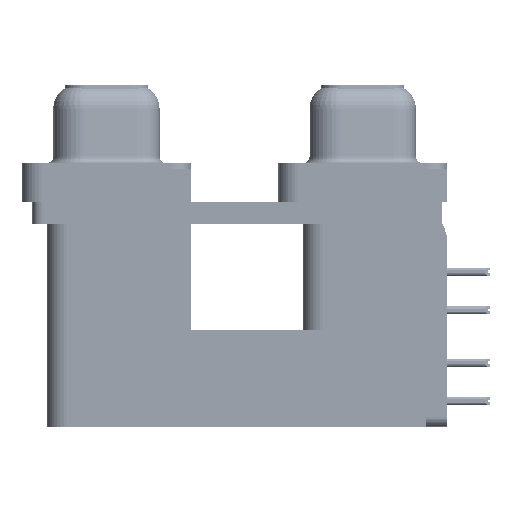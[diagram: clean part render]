
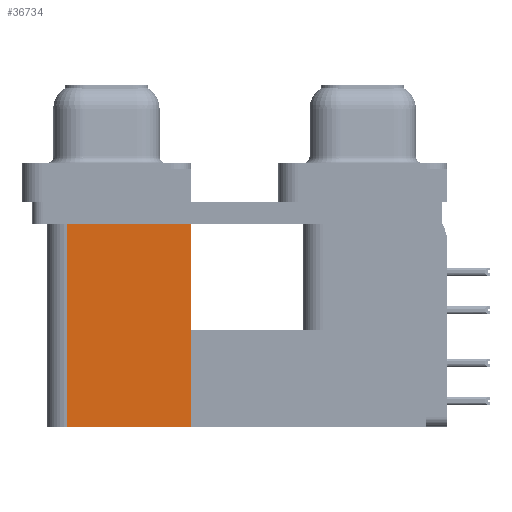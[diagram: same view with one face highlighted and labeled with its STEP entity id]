
A CAD part, left-side view. The second image highlights one B-rep face of the part: STEP entity #36734.
In plain terms, the highlighted planar face has unit normal (-1, 0, 0).
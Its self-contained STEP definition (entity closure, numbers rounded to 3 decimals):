
#5971 = LINE ( 'NONE', #34395, #34977 ) ;
#8221 = CARTESIAN_POINT ( 'NONE',  ( 3.7, 12.775, -19.2 ) ) ;
#8814 = EDGE_CURVE ( 'NONE', #12641, #12418, #5971, .T. ) ;
#10462 = VECTOR ( 'NONE', #11868, 1000. ) ;
#11868 = DIRECTION ( 'NONE',  ( 0., 1., 0. ) ) ;
#12096 = ORIENTED_EDGE ( 'NONE', *, *, #24958, .T. ) ;
#12418 = VERTEX_POINT ( 'NONE', #20148 ) ;
#12641 = VERTEX_POINT ( 'NONE', #27373 ) ;
#16470 = LINE ( 'NONE', #35119, #10462 ) ;
#20148 = CARTESIAN_POINT ( 'NONE',  ( 3.7, 21.975, -19.2 ) ) ;
#20913 = FACE_OUTER_BOUND ( 'NONE', #24763, .T. ) ;
#23416 = CARTESIAN_POINT ( 'NONE',  ( 3.7, 21.975, -19.2 ) ) ;
#24763 = EDGE_LOOP ( 'NONE', ( #60352, #52132, #34953, #12096 ) ) ;
#24958 = EDGE_CURVE ( 'NONE', #12641, #39549, #32352, .T. ) ;
#27373 = CARTESIAN_POINT ( 'NONE',  ( 3.7, 12.775, -19.2 ) ) ;
#31289 = DIRECTION ( 'NONE',  ( 0., 1., 0. ) ) ;
#32352 = LINE ( 'NONE', #8221, #49107 ) ;
#32869 = VECTOR ( 'NONE', #41470, 1000. ) ;
#33823 = AXIS2_PLACEMENT_3D ( 'NONE', #39895, #44779, #31289 ) ;
#34395 = CARTESIAN_POINT ( 'NONE',  ( 3.7, 12.775, -19.2 ) ) ;
#34953 = ORIENTED_EDGE ( 'NONE', *, *, #8814, .F. ) ;
#34977 = VECTOR ( 'NONE', #53071, 1000. ) ;
#35119 = CARTESIAN_POINT ( 'NONE',  ( 3.7, 12.775, -2.5 ) ) ;
#36567 = LINE ( 'NONE', #23416, #32869 ) ;
#36734 = ADVANCED_FACE ( 'NONE', ( #20913 ), #53355, .F. ) ;
#37438 = EDGE_CURVE ( 'NONE', #12418, #55765, #36567, .T. ) ;
#39549 = VERTEX_POINT ( 'NONE', #43365 ) ;
#39895 = CARTESIAN_POINT ( 'NONE',  ( 3.7, 12.775, -19.2 ) ) ;
#41470 = DIRECTION ( 'NONE',  ( 0., 0., 1. ) ) ;
#43365 = CARTESIAN_POINT ( 'NONE',  ( 3.7, 12.775, -2.5 ) ) ;
#44779 = DIRECTION ( 'NONE',  ( 1., 0., 0. ) ) ;
#48243 = CARTESIAN_POINT ( 'NONE',  ( 3.7, 21.975, -2.5 ) ) ;
#49107 = VECTOR ( 'NONE', #50741, 1000. ) ;
#50741 = DIRECTION ( 'NONE',  ( 0., 0., 1. ) ) ;
#52132 = ORIENTED_EDGE ( 'NONE', *, *, #37438, .F. ) ;
#53071 = DIRECTION ( 'NONE',  ( 0., 1., 0. ) ) ;
#53355 = PLANE ( 'NONE',  #33823 ) ;
#54096 = EDGE_CURVE ( 'NONE', #39549, #55765, #16470, .T. ) ;
#55765 = VERTEX_POINT ( 'NONE', #48243 ) ;
#60352 = ORIENTED_EDGE ( 'NONE', *, *, #54096, .T. ) ;
